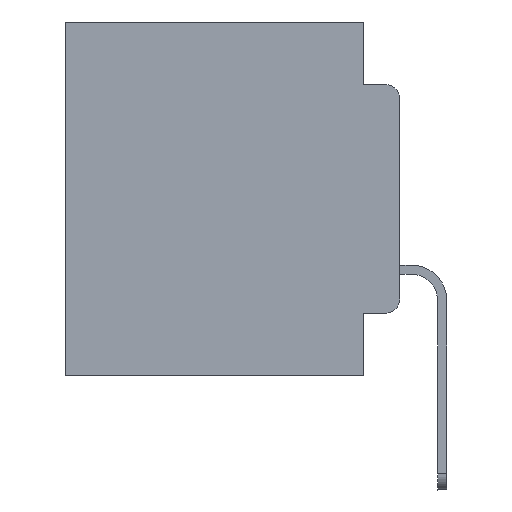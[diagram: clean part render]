
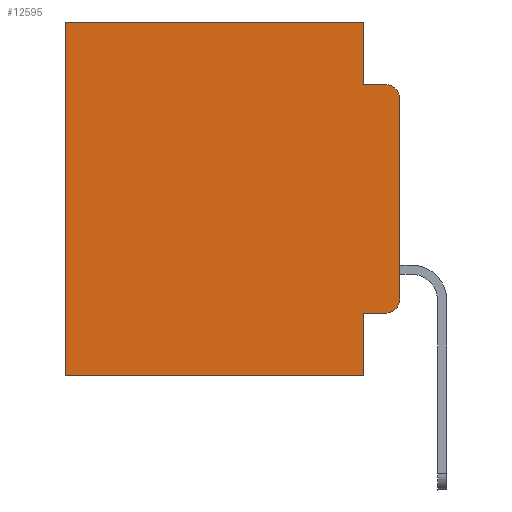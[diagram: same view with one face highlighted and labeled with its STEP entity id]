
A CAD part, left-side view. The second image highlights one B-rep face of the part: STEP entity #12595.
In plain terms, the highlighted planar face has unit normal (-1, 0, 0).
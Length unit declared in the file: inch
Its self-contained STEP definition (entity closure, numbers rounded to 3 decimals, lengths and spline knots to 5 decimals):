
#41 = VERTEX_POINT ( 'NONE', #23899 ) ;
#310 = PLANE ( 'NONE',  #9354 ) ;
#706 = VERTEX_POINT ( 'NONE', #8232 ) ;
#708 = CARTESIAN_POINT ( 'NONE',  ( 0.298, 0., 0. ) ) ;
#1083 = CARTESIAN_POINT ( 'NONE',  ( 0.298, 0., -0.5 ) ) ;
#1846 = ORIENTED_EDGE ( 'NONE', *, *, #11429, .F. ) ;
#1975 = CARTESIAN_POINT ( 'NONE',  ( 0.298, 0.051, 0. ) ) ;
#2556 = CARTESIAN_POINT ( 'NONE',  ( 0.298, 0., 0. ) ) ;
#3101 = EDGE_CURVE ( 'NONE', #41, #18362, #15110, .T. ) ;
#3125 = LINE ( 'NONE', #1083, #3627 ) ;
#3146 = AXIS2_PLACEMENT_3D ( 'NONE', #13510, #21860, #20207 ) ;
#3627 = VECTOR ( 'NONE', #13390, 39.37008 ) ;
#3753 = VECTOR ( 'NONE', #25286, 39.37008 ) ;
#4350 = DIRECTION ( 'NONE',  ( 0., 0., -1. ) ) ;
#4450 = CARTESIAN_POINT ( 'NONE',  ( 0.298, 0.02, -0.0885 ) ) ;
#4721 = CARTESIAN_POINT ( 'NONE',  ( 0.298, 0.051, -0.4115 ) ) ;
#4768 = DIRECTION ( 'NONE',  ( -1., 0., 0. ) ) ;
#5586 = CARTESIAN_POINT ( 'NONE',  ( 0.298, 0., -0.3915 ) ) ;
#5637 = VECTOR ( 'NONE', #17025, 39.37008 ) ;
#5950 = ORIENTED_EDGE ( 'NONE', *, *, #9085, .T. ) ;
#5975 = DIRECTION ( 'NONE',  ( 0., -1., 0. ) ) ;
#6202 = VECTOR ( 'NONE', #5975, 39.37008 ) ;
#7167 = VERTEX_POINT ( 'NONE', #16847 ) ;
#7373 = CARTESIAN_POINT ( 'NONE',  ( 0.298, 0., -0.1085 ) ) ;
#7525 = ORIENTED_EDGE ( 'NONE', *, *, #21096, .T. ) ;
#7903 = VECTOR ( 'NONE', #26063, 39.37008 ) ;
#8232 = CARTESIAN_POINT ( 'NONE',  ( 0.298, 0.02, -0.4115 ) ) ;
#8402 = VERTEX_POINT ( 'NONE', #1975 ) ;
#8427 = ORIENTED_EDGE ( 'NONE', *, *, #8915, .T. ) ;
#8642 = DIRECTION ( 'NONE',  ( 1., 0., 0. ) ) ;
#8915 = EDGE_CURVE ( 'NONE', #706, #13179, #11856, .T. ) ;
#9085 = EDGE_CURVE ( 'NONE', #24191, #19664, #24541, .T. ) ;
#9237 = EDGE_CURVE ( 'NONE', #23165, #19664, #20475, .T. ) ;
#9354 = AXIS2_PLACEMENT_3D ( 'NONE', #26844, #8642, #16989 ) ;
#10313 = ORIENTED_EDGE ( 'NONE', *, *, #10320, .T. ) ;
#10320 = EDGE_CURVE ( 'NONE', #8402, #41, #22030, .T. ) ;
#10691 = FACE_OUTER_BOUND ( 'NONE', #26008, .T. ) ;
#11092 = CARTESIAN_POINT ( 'NONE',  ( 0.298, 0.051, 0. ) ) ;
#11229 = LINE ( 'NONE', #11092, #22028 ) ;
#11429 = EDGE_CURVE ( 'NONE', #8402, #23165, #11229, .T. ) ;
#11856 = CIRCLE ( 'NONE', #12729, 0.02 ) ;
#12255 = CARTESIAN_POINT ( 'NONE',  ( 0.298, 0.051, -0.4115 ) ) ;
#12371 = VECTOR ( 'NONE', #13676, 39.37008 ) ;
#12595 = ADVANCED_FACE ( 'NONE', ( #10691 ), #310, .F. ) ;
#12729 = AXIS2_PLACEMENT_3D ( 'NONE', #21310, #4768, #15292 ) ;
#13179 = VERTEX_POINT ( 'NONE', #5586 ) ;
#13390 = DIRECTION ( 'NONE',  ( 0., 1., 0. ) ) ;
#13510 = CARTESIAN_POINT ( 'NONE',  ( 0.298, 0.02, -0.1085 ) ) ;
#13676 = DIRECTION ( 'NONE',  ( 0., 1., 0. ) ) ;
#14583 = ORIENTED_EDGE ( 'NONE', *, *, #22903, .F. ) ;
#14702 = CARTESIAN_POINT ( 'NONE',  ( 0.298, 0.473, 0. ) ) ;
#15110 = LINE ( 'NONE', #14702, #5637 ) ;
#15292 = DIRECTION ( 'NONE',  ( 0., 0., -1. ) ) ;
#16644 = ORIENTED_EDGE ( 'NONE', *, *, #9237, .F. ) ;
#16795 = CARTESIAN_POINT ( 'NONE',  ( 0.298, 0.051, -0.0885 ) ) ;
#16847 = CARTESIAN_POINT ( 'NONE',  ( 0.298, 0.051, -0.5 ) ) ;
#16989 = DIRECTION ( 'NONE',  ( 0., 0., -1. ) ) ;
#17025 = DIRECTION ( 'NONE',  ( 0., 0., -1. ) ) ;
#17055 = ORIENTED_EDGE ( 'NONE', *, *, #24417, .F. ) ;
#17217 = CARTESIAN_POINT ( 'NONE',  ( 0.298, 0.051, 0. ) ) ;
#17963 = EDGE_CURVE ( 'NONE', #18345, #7167, #21183, .T. ) ;
#18028 = CARTESIAN_POINT ( 'NONE',  ( 0.298, 0.473, -0.5 ) ) ;
#18345 = VERTEX_POINT ( 'NONE', #12255 ) ;
#18362 = VERTEX_POINT ( 'NONE', #18028 ) ;
#19105 = LINE ( 'NONE', #2556, #25964 ) ;
#19443 = DIRECTION ( 'NONE',  ( 0., 0., -1. ) ) ;
#19664 = VERTEX_POINT ( 'NONE', #4450 ) ;
#20207 = DIRECTION ( 'NONE',  ( 0., 0., -1. ) ) ;
#20475 = LINE ( 'NONE', #24722, #6202 ) ;
#21096 = EDGE_CURVE ( 'NONE', #18345, #706, #23605, .T. ) ;
#21150 = ORIENTED_EDGE ( 'NONE', *, *, #3101, .T. ) ;
#21183 = LINE ( 'NONE', #17217, #3753 ) ;
#21310 = CARTESIAN_POINT ( 'NONE',  ( 0.298, 0.02, -0.3915 ) ) ;
#21860 = DIRECTION ( 'NONE',  ( -1., 0., 0. ) ) ;
#22028 = VECTOR ( 'NONE', #19443, 39.37008 ) ;
#22030 = LINE ( 'NONE', #708, #12371 ) ;
#22835 = ORIENTED_EDGE ( 'NONE', *, *, #17963, .F. ) ;
#22903 = EDGE_CURVE ( 'NONE', #7167, #18362, #3125, .T. ) ;
#23165 = VERTEX_POINT ( 'NONE', #16795 ) ;
#23605 = LINE ( 'NONE', #4721, #7903 ) ;
#23899 = CARTESIAN_POINT ( 'NONE',  ( 0.298, 0.473, 0. ) ) ;
#24191 = VERTEX_POINT ( 'NONE', #7373 ) ;
#24417 = EDGE_CURVE ( 'NONE', #24191, #13179, #19105, .T. ) ;
#24541 = CIRCLE ( 'NONE', #3146, 0.02 ) ;
#24722 = CARTESIAN_POINT ( 'NONE',  ( 0.298, 0.051, -0.0885 ) ) ;
#25286 = DIRECTION ( 'NONE',  ( 0., 0., -1. ) ) ;
#25964 = VECTOR ( 'NONE', #4350, 39.37008 ) ;
#26008 = EDGE_LOOP ( 'NONE', ( #17055, #5950, #16644, #1846, #10313, #21150, #14583, #22835, #7525, #8427 ) ) ;
#26063 = DIRECTION ( 'NONE',  ( 0., -1., 0. ) ) ;
#26844 = CARTESIAN_POINT ( 'NONE',  ( 0.298, 0., 0. ) ) ;
